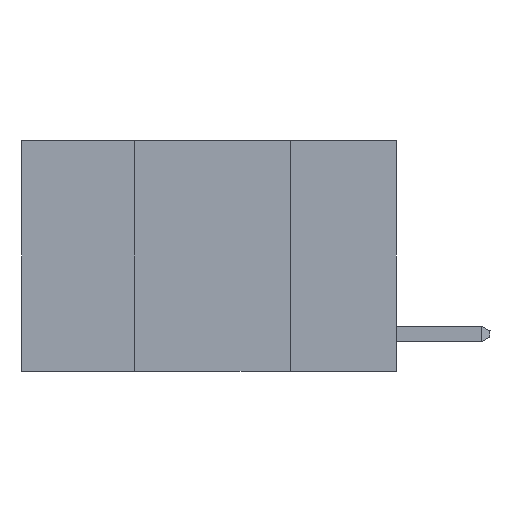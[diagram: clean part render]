
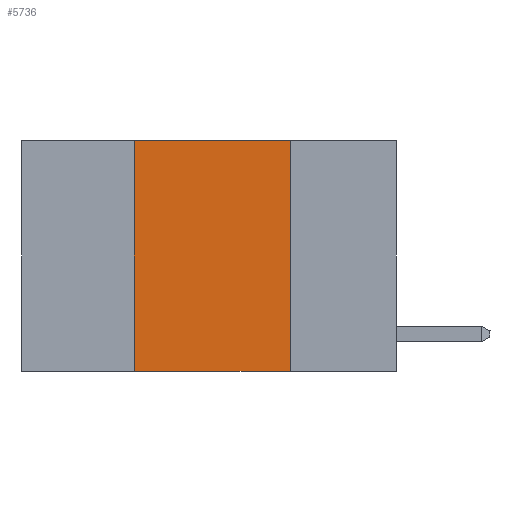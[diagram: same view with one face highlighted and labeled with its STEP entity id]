
A CAD part, left-side view. The second image highlights one B-rep face of the part: STEP entity #5736.
In plain terms, the highlighted planar face has unit normal (-1, 0, 0).
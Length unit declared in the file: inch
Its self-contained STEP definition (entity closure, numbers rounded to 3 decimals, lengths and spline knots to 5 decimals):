
#360 = CARTESIAN_POINT ( 'NONE',  ( 0., 0.42, -0.37 ) ) ;
#703 = VERTEX_POINT ( 'NONE', #360 ) ;
#2875 = ORIENTED_EDGE ( 'NONE', *, *, #7753, .T. ) ;
#2924 = DIRECTION ( 'NONE',  ( 1., 0., 0. ) ) ;
#2955 = AXIS2_PLACEMENT_3D ( 'NONE', #8888, #2924, #13722 ) ;
#3269 = CARTESIAN_POINT ( 'NONE',  ( 0., 0.42, 0. ) ) ;
#3353 = CARTESIAN_POINT ( 'NONE',  ( 0., 0.17, 0. ) ) ;
#3356 = EDGE_CURVE ( 'NONE', #13592, #5372, #6756, .T. ) ;
#3916 = PLANE ( 'NONE',  #2955 ) ;
#4528 = CARTESIAN_POINT ( 'NONE',  ( 0., 0.6, -0.37 ) ) ;
#5183 = DIRECTION ( 'NONE',  ( 0., 0., -1. ) ) ;
#5222 = ORIENTED_EDGE ( 'NONE', *, *, #7763, .F. ) ;
#5362 = CARTESIAN_POINT ( 'NONE',  ( 0., 0.17, -0.37 ) ) ;
#5372 = VERTEX_POINT ( 'NONE', #12721 ) ;
#5736 = ADVANCED_FACE ( 'NONE', ( #14115 ), #3916, .F. ) ;
#5850 = LINE ( 'NONE', #6990, #14996 ) ;
#6756 = LINE ( 'NONE', #8643, #9564 ) ;
#6838 = DIRECTION ( 'NONE',  ( 0., -1., 0. ) ) ;
#6990 = CARTESIAN_POINT ( 'NONE',  ( 0., 0.42, 0. ) ) ;
#7320 = ORIENTED_EDGE ( 'NONE', *, *, #3356, .F. ) ;
#7753 = EDGE_CURVE ( 'NONE', #703, #13926, #12761, .T. ) ;
#7763 = EDGE_CURVE ( 'NONE', #703, #13592, #5850, .T. ) ;
#8244 = EDGE_CURVE ( 'NONE', #5372, #13926, #9398, .T. ) ;
#8643 = CARTESIAN_POINT ( 'NONE',  ( 0., 0.6, 0. ) ) ;
#8888 = CARTESIAN_POINT ( 'NONE',  ( 0., 0.6, 0. ) ) ;
#8980 = VECTOR ( 'NONE', #5183, 39.37008 ) ;
#9398 = LINE ( 'NONE', #3353, #8980 ) ;
#9564 = VECTOR ( 'NONE', #13327, 39.37008 ) ;
#11111 = ORIENTED_EDGE ( 'NONE', *, *, #8244, .F. ) ;
#12094 = EDGE_LOOP ( 'NONE', ( #11111, #7320, #5222, #2875 ) ) ;
#12721 = CARTESIAN_POINT ( 'NONE',  ( 0., 0.17, 0. ) ) ;
#12736 = DIRECTION ( 'NONE',  ( 0., 0., 1. ) ) ;
#12761 = LINE ( 'NONE', #4528, #14048 ) ;
#13327 = DIRECTION ( 'NONE',  ( 0., -1., 0. ) ) ;
#13592 = VERTEX_POINT ( 'NONE', #3269 ) ;
#13722 = DIRECTION ( 'NONE',  ( 0., 0., -1. ) ) ;
#13926 = VERTEX_POINT ( 'NONE', #5362 ) ;
#14048 = VECTOR ( 'NONE', #6838, 39.37008 ) ;
#14115 = FACE_OUTER_BOUND ( 'NONE', #12094, .T. ) ;
#14996 = VECTOR ( 'NONE', #12736, 39.37008 ) ;
